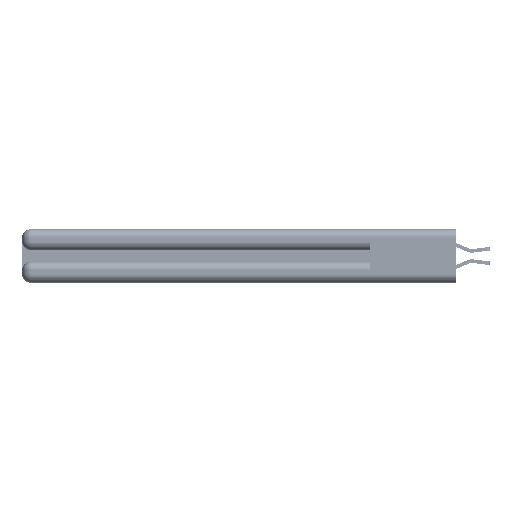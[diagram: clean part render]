
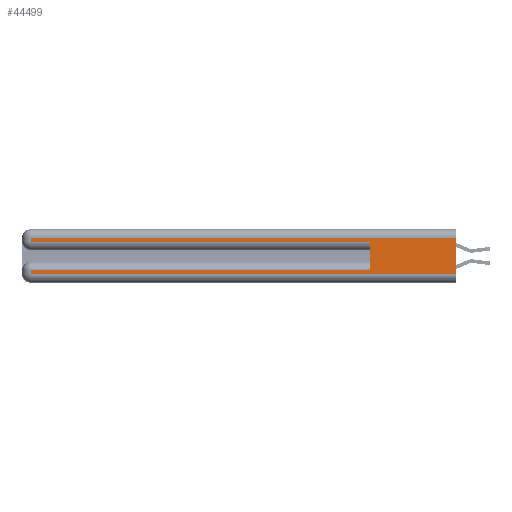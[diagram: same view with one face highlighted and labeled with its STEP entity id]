
A CAD part, left-side view. The second image highlights one B-rep face of the part: STEP entity #44499.
In plain terms, the highlighted planar face has unit normal (-1, 0, 0).
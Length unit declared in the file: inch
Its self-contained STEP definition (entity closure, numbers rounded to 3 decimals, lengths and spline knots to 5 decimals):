
#100 = EDGE_CURVE ( 'NONE', #42190, #13497, #33911, .T. ) ;
#671 = DIRECTION ( 'NONE',  ( 0., 0., -1. ) ) ;
#692 = CARTESIAN_POINT ( 'NONE',  ( 0., 0., 0.285 ) ) ;
#2568 = LINE ( 'NONE', #39094, #9852 ) ;
#2670 = ORIENTED_EDGE ( 'NONE', *, *, #7858, .F. ) ;
#3176 = FACE_OUTER_BOUND ( 'NONE', #33543, .T. ) ;
#3231 = LINE ( 'NONE', #692, #23063 ) ;
#3622 = EDGE_CURVE ( 'NONE', #30154, #31640, #2568, .T. ) ;
#4930 = LINE ( 'NONE', #40757, #8872 ) ;
#5631 = CARTESIAN_POINT ( 'NONE',  ( 0., 0., 0.37 ) ) ;
#5767 = DIRECTION ( 'NONE',  ( 0., 0., -1. ) ) ;
#6228 = AXIS2_PLACEMENT_3D ( 'NONE', #29831, #44421, #671 ) ;
#7063 = CARTESIAN_POINT ( 'NONE',  ( 0., 2.94, 0.285 ) ) ;
#7858 = EDGE_CURVE ( 'NONE', #42190, #31640, #45846, .T. ) ;
#8065 = EDGE_CURVE ( 'NONE', #41969, #13018, #4930, .T. ) ;
#8872 = VECTOR ( 'NONE', #37768, 39.37008 ) ;
#9546 = LINE ( 'NONE', #21517, #27725 ) ;
#9852 = VECTOR ( 'NONE', #33424, 39.37008 ) ;
#12511 = EDGE_CURVE ( 'NONE', #13018, #30154, #30896, .T. ) ;
#13018 = VERTEX_POINT ( 'NONE', #25348 ) ;
#13497 = VERTEX_POINT ( 'NONE', #40563 ) ;
#15120 = VECTOR ( 'NONE', #20191, 39.37008 ) ;
#15377 = ORIENTED_EDGE ( 'NONE', *, *, #8065, .T. ) ;
#15775 = DIRECTION ( 'NONE',  ( 0., 1., 0. ) ) ;
#16279 = CARTESIAN_POINT ( 'NONE',  ( 0., 2.94, 0.37 ) ) ;
#16437 = CARTESIAN_POINT ( 'NONE',  ( 0., 0.6, 0.085 ) ) ;
#18000 = EDGE_CURVE ( 'NONE', #41969, #23021, #9546, .T. ) ;
#18109 = ORIENTED_EDGE ( 'NONE', *, *, #18000, .F. ) ;
#20191 = DIRECTION ( 'NONE',  ( 0., 0., -1. ) ) ;
#20524 = CARTESIAN_POINT ( 'NONE',  ( 0., 2.94, 0.06 ) ) ;
#20742 = EDGE_CURVE ( 'NONE', #13497, #24664, #25784, .T. ) ;
#21073 = ORIENTED_EDGE ( 'NONE', *, *, #100, .T. ) ;
#21517 = CARTESIAN_POINT ( 'NONE',  ( 0., 0.6, 0.145 ) ) ;
#23021 = VERTEX_POINT ( 'NONE', #27223 ) ;
#23063 = VECTOR ( 'NONE', #37164, 39.37008 ) ;
#23409 = EDGE_CURVE ( 'NONE', #24664, #23021, #3231, .T. ) ;
#23536 = ORIENTED_EDGE ( 'NONE', *, *, #20742, .T. ) ;
#24099 = DIRECTION ( 'NONE',  ( 0., 0., 1. ) ) ;
#24359 = ORIENTED_EDGE ( 'NONE', *, *, #23409, .T. ) ;
#24664 = VERTEX_POINT ( 'NONE', #7063 ) ;
#25348 = CARTESIAN_POINT ( 'NONE',  ( 0., 2.94, 0.085 ) ) ;
#25784 = LINE ( 'NONE', #16279, #42862 ) ;
#26755 = ORIENTED_EDGE ( 'NONE', *, *, #12511, .T. ) ;
#27223 = CARTESIAN_POINT ( 'NONE',  ( 0., 0.6, 0.285 ) ) ;
#27725 = VECTOR ( 'NONE', #24099, 39.37008 ) ;
#27839 = CARTESIAN_POINT ( 'NONE',  ( 0., 0., 0.06 ) ) ;
#28035 = CARTESIAN_POINT ( 'NONE',  ( 0., 0., 0.31 ) ) ;
#28040 = DIRECTION ( 'NONE',  ( 0., 0., -1. ) ) ;
#29831 = CARTESIAN_POINT ( 'NONE',  ( 0., 0., 0.37 ) ) ;
#30154 = VERTEX_POINT ( 'NONE', #20524 ) ;
#30896 = LINE ( 'NONE', #45600, #37743 ) ;
#31640 = VERTEX_POINT ( 'NONE', #27839 ) ;
#33329 = VECTOR ( 'NONE', #15775, 39.37008 ) ;
#33424 = DIRECTION ( 'NONE',  ( 0., -1., 0. ) ) ;
#33543 = EDGE_LOOP ( 'NONE', ( #2670, #21073, #23536, #24359, #18109, #15377, #26755, #40355 ) ) ;
#33911 = LINE ( 'NONE', #34188, #33329 ) ;
#34188 = CARTESIAN_POINT ( 'NONE',  ( 0., 0., 0.31 ) ) ;
#37164 = DIRECTION ( 'NONE',  ( 0., -1., 0. ) ) ;
#37627 = PLANE ( 'NONE',  #6228 ) ;
#37743 = VECTOR ( 'NONE', #5767, 39.37008 ) ;
#37768 = DIRECTION ( 'NONE',  ( 0., 1., 0. ) ) ;
#39094 = CARTESIAN_POINT ( 'NONE',  ( 0., 0., 0.06 ) ) ;
#40355 = ORIENTED_EDGE ( 'NONE', *, *, #3622, .T. ) ;
#40563 = CARTESIAN_POINT ( 'NONE',  ( 0., 2.94, 0.31 ) ) ;
#40757 = CARTESIAN_POINT ( 'NONE',  ( 0., 0., 0.085 ) ) ;
#41969 = VERTEX_POINT ( 'NONE', #16437 ) ;
#42190 = VERTEX_POINT ( 'NONE', #28035 ) ;
#42862 = VECTOR ( 'NONE', #28040, 39.37008 ) ;
#44421 = DIRECTION ( 'NONE',  ( 1., 0., 0. ) ) ;
#44499 = ADVANCED_FACE ( 'NONE', ( #3176 ), #37627, .F. ) ;
#45600 = CARTESIAN_POINT ( 'NONE',  ( 0., 2.94, 0.37 ) ) ;
#45846 = LINE ( 'NONE', #5631, #15120 ) ;
